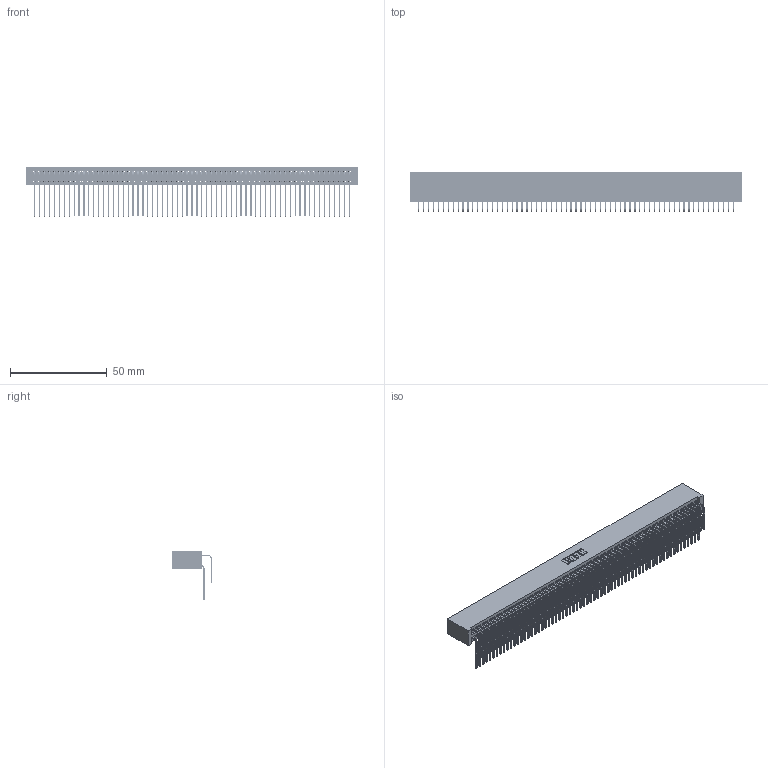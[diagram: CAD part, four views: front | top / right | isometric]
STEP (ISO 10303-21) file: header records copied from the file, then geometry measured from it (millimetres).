
FILE_DESCRIPTION (( 'STEP AP203' ), '1' );
FILE_NAME ('395-130-559-201.STEP', '2018-12-04T19:51:39', ( '' ), ( '' ), 'SwSTEP 2.0', 'SolidWorks 2016', '' );
FILE_SCHEMA (( 'CONFIG_CONTROL_DESIGN' ));
Length unit declared in the file: inch
Products named in the file (4): 395-130-559-201; 345-292-001_558 559 Tail - 1; 345-292-001_559 Tail - 2; 345 Part_No Mounting Lugs
Assembly tree (131 placements, depth 2):
  395-130-559-201
    345 Part_No Mounting Lugs
    345-292-001_558 559 Tail - 1  x65
    345-292-001_559 Tail - 2  x65
Bounding box: 171.7 x 20.56 x 25.53 mm (x, y, z)
Volume: 18258.8 mm3; surface area: 31264.8 mm2
Topology: 131 solids, 131 shells, 6878 faces, 20467 edges, 13470 vertices
Faces by surface type: plane 4626, cylinder 2252
Entity records: 49279 total; most frequent: CARTESIAN_POINT 8283, ORIENTED_EDGE 8166, DIRECTION 7243, EDGE_CURVE 4083, LINE 3659, VECTOR 3659, VERTEX_POINT 2718, AXIS2_PLACEMENT_3D 1792
